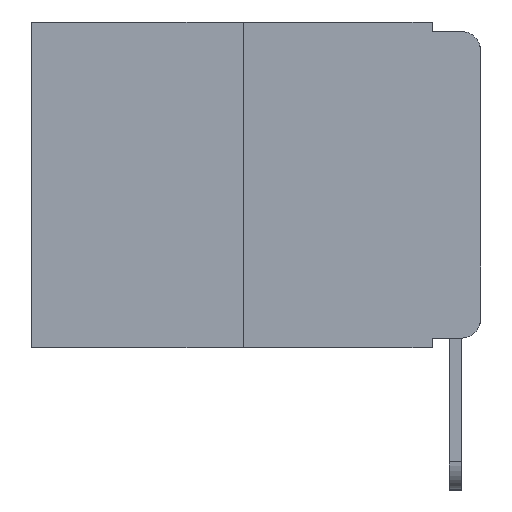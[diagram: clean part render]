
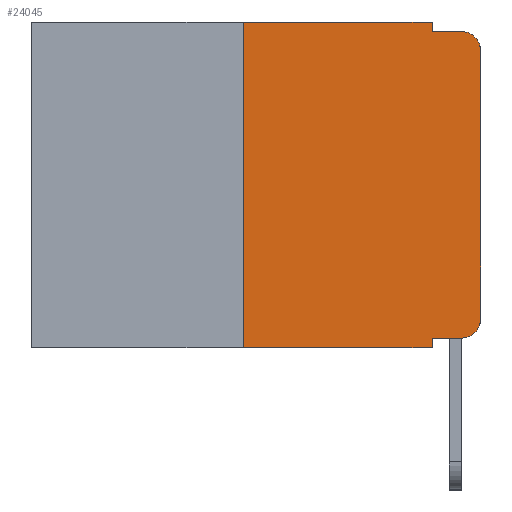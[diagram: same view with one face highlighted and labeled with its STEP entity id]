
A CAD part, left-side view. The second image highlights one B-rep face of the part: STEP entity #24045.
In plain terms, the highlighted planar face has unit normal (-1, 0, 0).
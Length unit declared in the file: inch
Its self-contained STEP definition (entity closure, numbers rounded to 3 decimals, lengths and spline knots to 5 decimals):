
#104 = VECTOR ( 'NONE', #19148, 39.37008 ) ;
#169 = CARTESIAN_POINT ( 'NONE',  ( 0., 0., 0. ) ) ;
#301 = EDGE_CURVE ( 'NONE', #10212, #16731, #14878, .T. ) ;
#343 = ORIENTED_EDGE ( 'NONE', *, *, #600, .T. ) ;
#346 = EDGE_CURVE ( 'NONE', #9854, #22222, #2775, .T. ) ;
#445 = EDGE_CURVE ( 'NONE', #1625, #7921, #11373, .T. ) ;
#600 = EDGE_CURVE ( 'NONE', #22222, #16731, #24046, .T. ) ;
#710 = VECTOR ( 'NONE', #5403, 39.37008 ) ;
#813 = EDGE_CURVE ( 'NONE', #4137, #9854, #11654, .T. ) ;
#964 = EDGE_CURVE ( 'NONE', #22174, #7921, #16977, .T. ) ;
#1610 = LINE ( 'NONE', #18224, #6073 ) ;
#1625 = VERTEX_POINT ( 'NONE', #4500 ) ;
#1742 = DIRECTION ( 'NONE',  ( -1., 0., 0. ) ) ;
#1869 = CARTESIAN_POINT ( 'NONE',  ( 0., 0.051, 0. ) ) ;
#1995 = EDGE_CURVE ( 'NONE', #22174, #4137, #15396, .T. ) ;
#2240 = ORIENTED_EDGE ( 'NONE', *, *, #346, .T. ) ;
#2497 = AXIS2_PLACEMENT_3D ( 'NONE', #17149, #7727, #9636 ) ;
#2628 = CARTESIAN_POINT ( 'NONE',  ( 0., 0., -0.03 ) ) ;
#2694 = EDGE_CURVE ( 'NONE', #18430, #3052, #14773, .T. ) ;
#2775 = LINE ( 'NONE', #169, #3379 ) ;
#2892 = CARTESIAN_POINT ( 'NONE',  ( 0., 0.051, -0.343 ) ) ;
#2899 = DIRECTION ( 'NONE',  ( 0., 0., 1. ) ) ;
#3052 = VERTEX_POINT ( 'NONE', #9703 ) ;
#3379 = VECTOR ( 'NONE', #19288, 39.37008 ) ;
#3700 = DIRECTION ( 'NONE',  ( 0., 0., -1. ) ) ;
#4137 = VERTEX_POINT ( 'NONE', #9881 ) ;
#4500 = CARTESIAN_POINT ( 'NONE',  ( 0., 0.25, -0.343 ) ) ;
#5399 = LINE ( 'NONE', #1869, #19906 ) ;
#5403 = DIRECTION ( 'NONE',  ( 0., -1., 0. ) ) ;
#5477 = DIRECTION ( 'NONE',  ( 0., 0., -1. ) ) ;
#5746 = CARTESIAN_POINT ( 'NONE',  ( 0., 0.02, -0.01 ) ) ;
#6073 = VECTOR ( 'NONE', #2899, 39.37008 ) ;
#6136 = ORIENTED_EDGE ( 'NONE', *, *, #813, .T. ) ;
#6203 = AXIS2_PLACEMENT_3D ( 'NONE', #11461, #17015, #3700 ) ;
#7237 = CARTESIAN_POINT ( 'NONE',  ( 0., 0.051, -0.01 ) ) ;
#7727 = DIRECTION ( 'NONE',  ( -1., 0., 0. ) ) ;
#7921 = VERTEX_POINT ( 'NONE', #2892 ) ;
#9544 = DIRECTION ( 'NONE',  ( 0., -1., 0. ) ) ;
#9636 = DIRECTION ( 'NONE',  ( 0., 0., -1. ) ) ;
#9670 = CARTESIAN_POINT ( 'NONE',  ( 0., 0.473, 0. ) ) ;
#9703 = CARTESIAN_POINT ( 'NONE',  ( 0., 0.051, 0. ) ) ;
#9854 = VERTEX_POINT ( 'NONE', #16291 ) ;
#9881 = CARTESIAN_POINT ( 'NONE',  ( 0., 0.02, -0.333 ) ) ;
#10105 = CARTESIAN_POINT ( 'NONE',  ( 0., 0.051, -0.333 ) ) ;
#10212 = VERTEX_POINT ( 'NONE', #12145 ) ;
#11142 = DIRECTION ( 'NONE',  ( 0., 0., -1. ) ) ;
#11373 = LINE ( 'NONE', #21365, #104 ) ;
#11461 = CARTESIAN_POINT ( 'NONE',  ( 0., 0.473, 0. ) ) ;
#11654 = CIRCLE ( 'NONE', #2497, 0.02 ) ;
#11956 = ORIENTED_EDGE ( 'NONE', *, *, #445, .T. ) ;
#12005 = ORIENTED_EDGE ( 'NONE', *, *, #15922, .F. ) ;
#12145 = CARTESIAN_POINT ( 'NONE',  ( 0., 0.051, -0.01 ) ) ;
#14198 = CARTESIAN_POINT ( 'NONE',  ( 0., 0.051, 0. ) ) ;
#14773 = LINE ( 'NONE', #9670, #22755 ) ;
#14815 = VECTOR ( 'NONE', #9544, 39.37008 ) ;
#14878 = LINE ( 'NONE', #7237, #710 ) ;
#15303 = FACE_OUTER_BOUND ( 'NONE', #22691, .T. ) ;
#15396 = LINE ( 'NONE', #17300, #14815 ) ;
#15506 = ORIENTED_EDGE ( 'NONE', *, *, #964, .F. ) ;
#15583 = ORIENTED_EDGE ( 'NONE', *, *, #1995, .T. ) ;
#15922 = EDGE_CURVE ( 'NONE', #1625, #18430, #1610, .T. ) ;
#16291 = CARTESIAN_POINT ( 'NONE',  ( 0., 0., -0.313 ) ) ;
#16435 = ORIENTED_EDGE ( 'NONE', *, *, #20208, .F. ) ;
#16731 = VERTEX_POINT ( 'NONE', #5746 ) ;
#16977 = LINE ( 'NONE', #14198, #19348 ) ;
#17015 = DIRECTION ( 'NONE',  ( 1., 0., 0. ) ) ;
#17149 = CARTESIAN_POINT ( 'NONE',  ( 0., 0.02, -0.313 ) ) ;
#17300 = CARTESIAN_POINT ( 'NONE',  ( 0., 0.051, -0.333 ) ) ;
#18224 = CARTESIAN_POINT ( 'NONE',  ( 0., 0.25, 0. ) ) ;
#18430 = VERTEX_POINT ( 'NONE', #22956 ) ;
#19148 = DIRECTION ( 'NONE',  ( 0., -1., 0. ) ) ;
#19237 = DIRECTION ( 'NONE',  ( 0., -1., 0. ) ) ;
#19288 = DIRECTION ( 'NONE',  ( 0., 0., 1. ) ) ;
#19348 = VECTOR ( 'NONE', #23585, 39.37008 ) ;
#19906 = VECTOR ( 'NONE', #11142, 39.37008 ) ;
#20208 = EDGE_CURVE ( 'NONE', #3052, #10212, #5399, .T. ) ;
#20947 = ORIENTED_EDGE ( 'NONE', *, *, #301, .F. ) ;
#21365 = CARTESIAN_POINT ( 'NONE',  ( 0., 0.473, -0.343 ) ) ;
#21959 = AXIS2_PLACEMENT_3D ( 'NONE', #24449, #1742, #5477 ) ;
#22174 = VERTEX_POINT ( 'NONE', #10105 ) ;
#22222 = VERTEX_POINT ( 'NONE', #2628 ) ;
#22340 = ORIENTED_EDGE ( 'NONE', *, *, #2694, .F. ) ;
#22691 = EDGE_LOOP ( 'NONE', ( #2240, #343, #20947, #16435, #22340, #12005, #11956, #15506, #15583, #6136 ) ) ;
#22755 = VECTOR ( 'NONE', #19237, 39.37008 ) ;
#22846 = PLANE ( 'NONE',  #6203 ) ;
#22956 = CARTESIAN_POINT ( 'NONE',  ( 0., 0.25, 0. ) ) ;
#23585 = DIRECTION ( 'NONE',  ( 0., 0., -1. ) ) ;
#24045 = ADVANCED_FACE ( 'NONE', ( #15303 ), #22846, .F. ) ;
#24046 = CIRCLE ( 'NONE', #21959, 0.02 ) ;
#24449 = CARTESIAN_POINT ( 'NONE',  ( 0., 0.02, -0.03 ) ) ;
